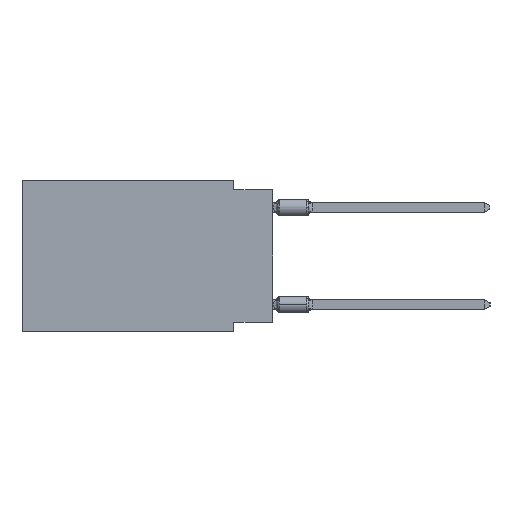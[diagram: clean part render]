
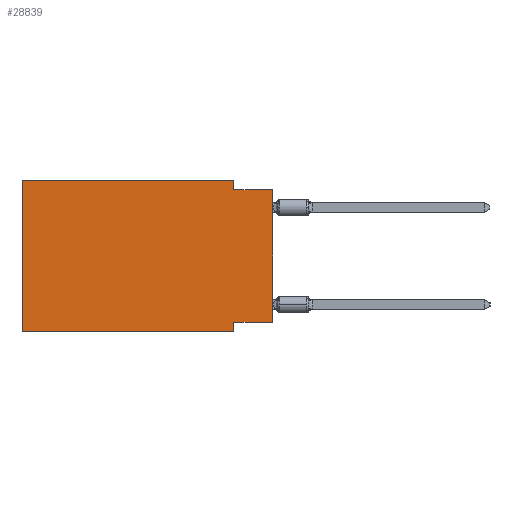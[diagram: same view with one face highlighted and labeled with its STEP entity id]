
A CAD part, left-side view. The second image highlights one B-rep face of the part: STEP entity #28839.
In plain terms, the highlighted planar face has unit normal (-1, 0, 0).
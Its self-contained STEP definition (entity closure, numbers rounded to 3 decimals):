
#642 = DIRECTION ( 'NONE',  ( 0., 0., -1. ) ) ;
#1640 = DIRECTION ( 'NONE',  ( 0., 0., -1. ) ) ;
#2719 = VERTEX_POINT ( 'NONE', #10317 ) ;
#3186 = EDGE_CURVE ( 'NONE', #35008, #11595, #15365, .T. ) ;
#3256 = DIRECTION ( 'NONE',  ( 0., -1., 0. ) ) ;
#4919 = CARTESIAN_POINT ( 'NONE',  ( 0., 2.54, -9.906 ) ) ;
#5774 = CARTESIAN_POINT ( 'NONE',  ( 0., 2.54, -9.271 ) ) ;
#5786 = DIRECTION ( 'NONE',  ( 0., -1., 0. ) ) ;
#6300 = CARTESIAN_POINT ( 'NONE',  ( 0., 2.54, -0.635 ) ) ;
#6668 = FACE_OUTER_BOUND ( 'NONE', #38150, .T. ) ;
#6754 = CARTESIAN_POINT ( 'NONE',  ( 0., 16.383, 0. ) ) ;
#8124 = EDGE_CURVE ( 'NONE', #35008, #35452, #20833, .T. ) ;
#8628 = CARTESIAN_POINT ( 'NONE',  ( 0., 16.383, -9.906 ) ) ;
#10095 = PLANE ( 'NONE',  #27674 ) ;
#10251 = VECTOR ( 'NONE', #36044, 1000. ) ;
#10317 = CARTESIAN_POINT ( 'NONE',  ( 0., 0., -0.635 ) ) ;
#10393 = ORIENTED_EDGE ( 'NONE', *, *, #20091, .T. ) ;
#11595 = VERTEX_POINT ( 'NONE', #6754 ) ;
#11919 = CARTESIAN_POINT ( 'NONE',  ( 0., 2.54, 0. ) ) ;
#14293 = CARTESIAN_POINT ( 'NONE',  ( 0., 2.54, 0. ) ) ;
#14398 = VECTOR ( 'NONE', #28801, 1000. ) ;
#14548 = ORIENTED_EDGE ( 'NONE', *, *, #8124, .T. ) ;
#14861 = VECTOR ( 'NONE', #3256, 1000. ) ;
#15036 = VERTEX_POINT ( 'NONE', #29626 ) ;
#15365 = LINE ( 'NONE', #31228, #32523 ) ;
#16324 = CARTESIAN_POINT ( 'NONE',  ( 0., 0., -9.271 ) ) ;
#16386 = VECTOR ( 'NONE', #1640, 1000. ) ;
#16546 = EDGE_CURVE ( 'NONE', #35540, #35452, #35237, .T. ) ;
#16957 = CARTESIAN_POINT ( 'NONE',  ( 0., 16.383, 0. ) ) ;
#17627 = DIRECTION ( 'NONE',  ( 0., -1., 0. ) ) ;
#18658 = VERTEX_POINT ( 'NONE', #6300 ) ;
#18952 = CARTESIAN_POINT ( 'NONE',  ( 0., 2.54, -9.906 ) ) ;
#19417 = EDGE_CURVE ( 'NONE', #11595, #26917, #22506, .T. ) ;
#19465 = VECTOR ( 'NONE', #5786, 1000. ) ;
#20091 = EDGE_CURVE ( 'NONE', #15036, #2719, #28595, .T. ) ;
#20833 = LINE ( 'NONE', #33914, #26039 ) ;
#22506 = LINE ( 'NONE', #38366, #19465 ) ;
#25140 = ORIENTED_EDGE ( 'NONE', *, *, #35097, .F. ) ;
#25233 = ORIENTED_EDGE ( 'NONE', *, *, #3186, .F. ) ;
#25420 = EDGE_CURVE ( 'NONE', #18658, #2719, #42081, .T. ) ;
#25494 = ORIENTED_EDGE ( 'NONE', *, *, #16546, .F. ) ;
#26039 = VECTOR ( 'NONE', #17627, 1000. ) ;
#26184 = LINE ( 'NONE', #16324, #10251 ) ;
#26917 = VERTEX_POINT ( 'NONE', #11919 ) ;
#27674 = AXIS2_PLACEMENT_3D ( 'NONE', #16957, #30032, #642 ) ;
#28595 = LINE ( 'NONE', #35017, #35926 ) ;
#28801 = DIRECTION ( 'NONE',  ( 0., 0., -1. ) ) ;
#28839 = ADVANCED_FACE ( 'NONE', ( #6668 ), #10095, .F. ) ;
#29626 = CARTESIAN_POINT ( 'NONE',  ( 0., 0., -9.271 ) ) ;
#30032 = DIRECTION ( 'NONE',  ( 1., 0., 0. ) ) ;
#30400 = ORIENTED_EDGE ( 'NONE', *, *, #25420, .F. ) ;
#31228 = CARTESIAN_POINT ( 'NONE',  ( 0., 16.383, 0. ) ) ;
#31235 = LINE ( 'NONE', #14293, #16386 ) ;
#31917 = EDGE_CURVE ( 'NONE', #26917, #18658, #31235, .T. ) ;
#32022 = CARTESIAN_POINT ( 'NONE',  ( 0., 0., -0.635 ) ) ;
#32523 = VECTOR ( 'NONE', #34669, 1000. ) ;
#32799 = ORIENTED_EDGE ( 'NONE', *, *, #19417, .F. ) ;
#33873 = ORIENTED_EDGE ( 'NONE', *, *, #31917, .F. ) ;
#33914 = CARTESIAN_POINT ( 'NONE',  ( 0., 16.383, -9.906 ) ) ;
#34669 = DIRECTION ( 'NONE',  ( 0., 0., 1. ) ) ;
#35008 = VERTEX_POINT ( 'NONE', #8628 ) ;
#35017 = CARTESIAN_POINT ( 'NONE',  ( 0., 0., 0. ) ) ;
#35097 = EDGE_CURVE ( 'NONE', #15036, #35540, #26184, .T. ) ;
#35226 = DIRECTION ( 'NONE',  ( 0., 0., 1. ) ) ;
#35237 = LINE ( 'NONE', #18952, #14398 ) ;
#35452 = VERTEX_POINT ( 'NONE', #4919 ) ;
#35540 = VERTEX_POINT ( 'NONE', #5774 ) ;
#35926 = VECTOR ( 'NONE', #35226, 1000. ) ;
#36044 = DIRECTION ( 'NONE',  ( 0., 1., 0. ) ) ;
#38150 = EDGE_LOOP ( 'NONE', ( #10393, #30400, #33873, #32799, #25233, #14548, #25494, #25140 ) ) ;
#38366 = CARTESIAN_POINT ( 'NONE',  ( 0., 16.383, 0. ) ) ;
#42081 = LINE ( 'NONE', #32022, #14861 ) ;
